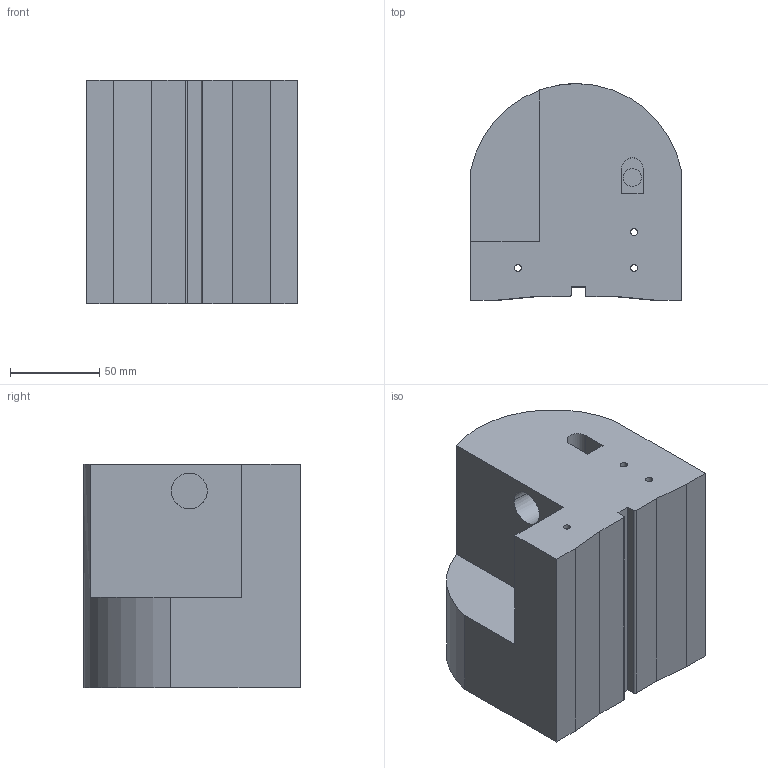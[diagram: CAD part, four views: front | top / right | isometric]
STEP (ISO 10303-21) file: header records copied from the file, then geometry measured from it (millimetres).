
FILE_DESCRIPTION (( 'STEP AP214' ), '1' );
FILE_NAME ('Normal Main Body Reciver.STEP', '2025-05-18T13:00:19', ( '' ), ( '' ), 'SwSTEP 2.0', 'SolidWorks 2024', '' );
FILE_SCHEMA (( 'AUTOMOTIVE_DESIGN' ));
Length unit declared in the file: millimetre
Products named in the file (1): Normal Main Body Reciver
Bounding box: 117.82 x 121 x 125 mm (x, y, z)
Volume: 1358085.4 mm3; surface area: 90879.1 mm2
Topology: 1 solids, 1 shells, 49 faces, 121 edges, 80 vertices
Faces by surface type: plane 26, cylinder 23
Entity records: 1645 total; most frequent: CARTESIAN_POINT 403, DIRECTION 260, ORIENTED_EDGE 242, EDGE_CURVE 121, AXIS2_PLACEMENT_3D 93, VERTEX_POINT 80, LINE 74, VECTOR 74
